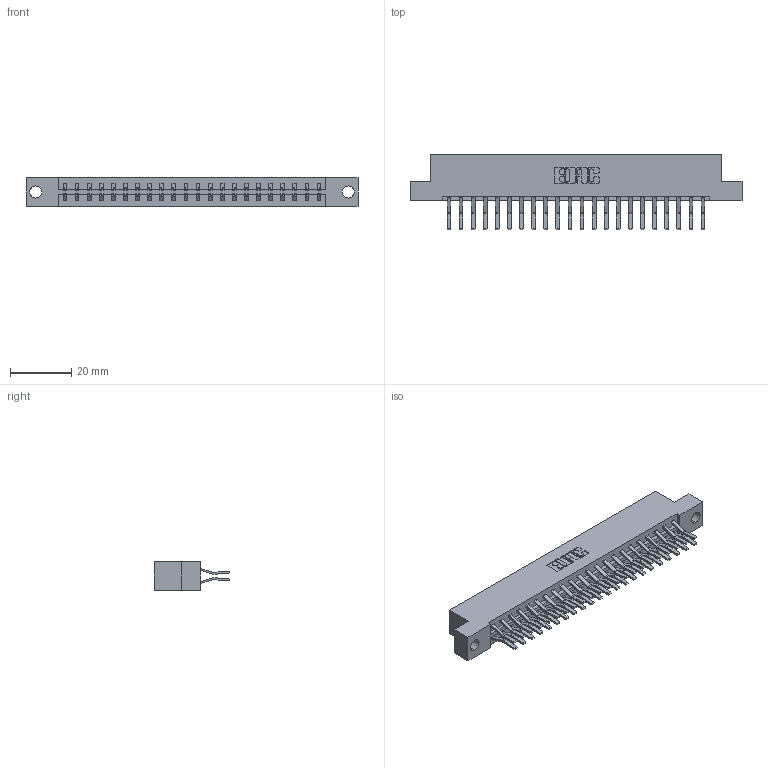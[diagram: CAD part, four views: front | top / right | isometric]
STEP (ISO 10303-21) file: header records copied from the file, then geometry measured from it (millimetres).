
FILE_DESCRIPTION (( 'STEP AP203' ), '1' );
FILE_NAME ('833-044-560-204.STEP', '2020-06-04T13:38:45', ( '' ), ( '' ), 'SwSTEP 2.0', 'SolidWorks 2020', '' );
FILE_SCHEMA (( 'CONFIG_CONTROL_DESIGN' ));
Length unit declared in the file: inch
Products named in the file (3): 345-292-001_560 Tail; 833-044-560-204; 833 Part_Flush - .156 Dia - TH
Assembly tree (45 placements, depth 2):
  833-044-560-204
    833 Part_Flush - .156 Dia - TH
    345-292-001_560 Tail  x44
Bounding box: 108.71 x 24.78 x 9.4 mm (x, y, z)
Volume: 11112.4 mm3; surface area: 13544.8 mm2
Topology: 45 solids, 45 shells, 2490 faces, 7395 edges, 4870 vertices
Faces by surface type: plane 1654, cylinder 836
Entity records: 16831 total; most frequent: CARTESIAN_POINT 2814, ORIENTED_EDGE 2750, DIRECTION 2443, EDGE_CURVE 1375, LINE 1243, VECTOR 1243, VERTEX_POINT 914, AXIS2_PLACEMENT_3D 600
